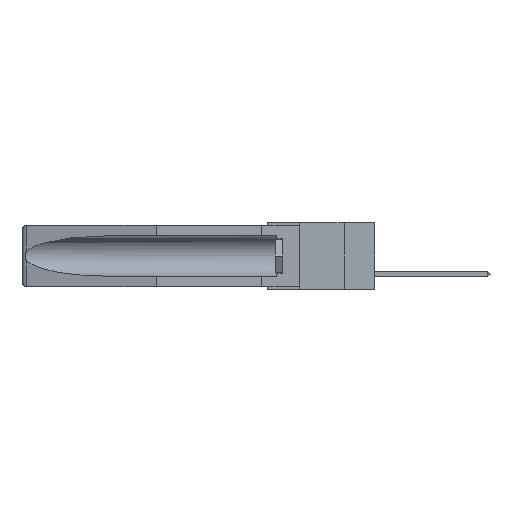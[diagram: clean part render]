
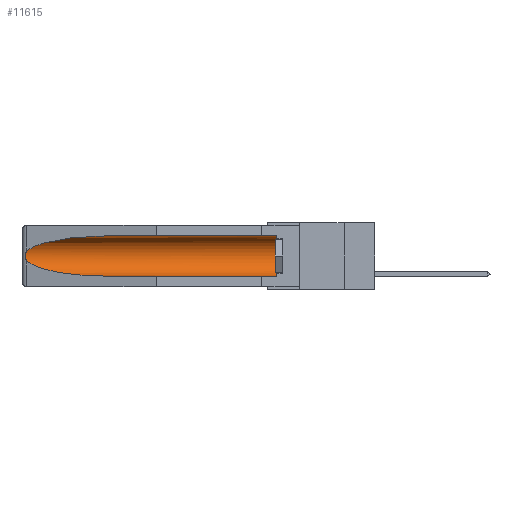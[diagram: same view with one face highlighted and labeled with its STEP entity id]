
A CAD part, left-side view. The second image highlights one B-rep face of the part: STEP entity #11615.
In plain terms, the highlighted cylindrical face has radius 2.857 mm (diameter 5.715 mm), a partial arc.
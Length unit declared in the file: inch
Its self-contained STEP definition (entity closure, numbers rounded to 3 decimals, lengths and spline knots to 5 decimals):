
#178 = AXIS2_PLACEMENT_3D ( 'NONE', #16693, #6734, #18355 ) ;
#640 = CARTESIAN_POINT ( 'NONE',  ( 0.26597, 1.5296, -0.19026 ) ) ;
#661 = CIRCLE ( 'NONE', #178, 0.1125 ) ;
#782 = CARTESIAN_POINT ( 'NONE',  ( 0.2673, 1.5327, -0.16383 ) ) ;
#856 = CARTESIAN_POINT ( 'NONE',  ( 0.2673, 1.53269, -0.17917 ) ) ;
#1087 = VERTEX_POINT ( 'NONE', #21462 ) ;
#1698 = CARTESIAN_POINT ( 'NONE',  ( 0.25451, 1.48313, -0.09465 ) ) ;
#1726 = EDGE_CURVE ( 'NONE', #5221, #7642, #12775, .T. ) ;
#2313 = CARTESIAN_POINT ( 'NONE',  ( 0.26654, 1.53092, -0.15636 ) ) ;
#3153 = ORIENTED_EDGE ( 'NONE', *, *, #1726, .T. ) ;
#3278 = EDGE_CURVE ( 'NONE', #10712, #8736, #7595, .T. ) ;
#3390 = ORIENTED_EDGE ( 'NONE', *, *, #7000, .F. ) ;
#3676 = EDGE_LOOP ( 'NONE', ( #18862, #15747, #3153, #3390, #4925, #5742 ) ) ;
#3760 = CARTESIAN_POINT ( 'NONE',  ( 0.155, -0.30754, -0.059 ) ) ;
#4052 = CARTESIAN_POINT ( 'NONE',  ( 0.25451, 1.48313, -0.24835 ) ) ;
#4061 = CARTESIAN_POINT ( 'NONE',  ( 0.2675, 1.53308, -0.17534 ) ) ;
#4267 = CARTESIAN_POINT ( 'NONE',  ( 0.21114, 1.30732, -0.284 ) ) ;
#4635 = EDGE_CURVE ( 'NONE', #11407, #1087, #661, .T. ) ;
#4812 = CARTESIAN_POINT ( 'NONE',  ( 0.26537, 1.52718, -0.14972 ) ) ;
#4925 = ORIENTED_EDGE ( 'NONE', *, *, #4635, .T. ) ;
#4960 = CARTESIAN_POINT ( 'NONE',  ( 0.21114, 1.30732, -0.059 ) ) ;
#5138 = LINE ( 'NONE', #3760, #9314 ) ;
#5221 = VERTEX_POINT ( 'NONE', #18161 ) ;
#5679 = CARTESIAN_POINT ( 'NONE',  ( 0.26537, 1.52718, -0.14972 ) ) ;
#5742 = ORIENTED_EDGE ( 'NONE', *, *, #10037, .T. ) ;
#5753 = CARTESIAN_POINT ( 'NONE',  ( 0.155, 0.126, -0.284 ) ) ;
#6734 = DIRECTION ( 'NONE',  ( 0., -1., 0. ) ) ;
#7000 = EDGE_CURVE ( 'NONE', #11407, #7642, #16149, .T. ) ;
#7356 = EDGE_CURVE ( 'NONE', #8736, #5221, #19863, .T. ) ;
#7595 =( BOUNDED_CURVE ( )  B_SPLINE_CURVE ( 3, ( #15014, #4960, #1698, #4812 ),
 .UNSPECIFIED., .F., .F. ) 
 B_SPLINE_CURVE_WITH_KNOTS ( ( 4, 4 ),
 ( 4.71239, 6.08839 ),
 .UNSPECIFIED. ) 
 CURVE ( )  GEOMETRIC_REPRESENTATION_ITEM ( )  RATIONAL_B_SPLINE_CURVE ( ( 1., 0.848, 0.848, 1. ) ) 
 REPRESENTATION_ITEM ( '' )  );
#7642 = VERTEX_POINT ( 'NONE', #20107 ) ;
#7922 = DIRECTION ( 'NONE',  ( 0., 0., 1. ) ) ;
#8483 = CYLINDRICAL_SURFACE ( 'NONE', #9733, 0.1125 ) ;
#8736 = VERTEX_POINT ( 'NONE', #5679 ) ;
#8780 = DIRECTION ( 'NONE',  ( 0., 1., 0. ) ) ;
#8874 = CARTESIAN_POINT ( 'NONE',  ( 0.26597, 1.52961, -0.15275 ) ) ;
#9314 = VECTOR ( 'NONE', #8780, 39.37008 ) ;
#9458 = DIRECTION ( 'NONE',  ( 0., 1., 0. ) ) ;
#9733 = AXIS2_PLACEMENT_3D ( 'NONE', #17867, #21228, #7922 ) ;
#10037 = EDGE_CURVE ( 'NONE', #1087, #10712, #5138, .T. ) ;
#10284 = FACE_OUTER_BOUND ( 'NONE', #3676, .T. ) ;
#10595 = CARTESIAN_POINT ( 'NONE',  ( 0.2675, 1.53308, -0.16763 ) ) ;
#10712 = VERTEX_POINT ( 'NONE', #12003 ) ;
#10804 = CARTESIAN_POINT ( 'NONE',  ( 0.26655, 1.53094, -0.18657 ) ) ;
#10825 = CARTESIAN_POINT ( 'NONE',  ( 0.155, -0.30754, -0.284 ) ) ;
#11407 = VERTEX_POINT ( 'NONE', #5753 ) ;
#11615 = ADVANCED_FACE ( 'NONE', ( #10284 ), #8483, .F. ) ;
#12003 = CARTESIAN_POINT ( 'NONE',  ( 0.155, 1.07973, -0.059 ) ) ;
#12764 = VECTOR ( 'NONE', #9458, 39.37008 ) ;
#12775 =( BOUNDED_CURVE ( )  B_SPLINE_CURVE ( 3, ( #17560, #4052, #4267, #17348 ),
 .UNSPECIFIED., .F., .T. ) 
 B_SPLINE_CURVE_WITH_KNOTS ( ( 4, 4 ),
 ( 0.1948, 1.5708 ),
 .UNSPECIFIED. ) 
 CURVE ( )  GEOMETRIC_REPRESENTATION_ITEM ( )  RATIONAL_B_SPLINE_CURVE ( ( 1., 0.848, 0.848, 1. ) ) 
 REPRESENTATION_ITEM ( '' )  );
#14088 = CARTESIAN_POINT ( 'NONE',  ( 0.26537, 1.52718, -0.19328 ) ) ;
#15014 = CARTESIAN_POINT ( 'NONE',  ( 0.155, 1.07973, -0.059 ) ) ;
#15641 = CARTESIAN_POINT ( 'NONE',  ( 0.26537, 1.52718, -0.14972 ) ) ;
#15747 = ORIENTED_EDGE ( 'NONE', *, *, #7356, .T. ) ;
#16149 = LINE ( 'NONE', #10825, #12764 ) ;
#16693 = CARTESIAN_POINT ( 'NONE',  ( 0.155, 0.126, -0.1715 ) ) ;
#17348 = CARTESIAN_POINT ( 'NONE',  ( 0.155, 1.07973, -0.284 ) ) ;
#17560 = CARTESIAN_POINT ( 'NONE',  ( 0.26537, 1.52718, -0.19328 ) ) ;
#17867 = CARTESIAN_POINT ( 'NONE',  ( 0.155, -0.30754, -0.1715 ) ) ;
#18161 = CARTESIAN_POINT ( 'NONE',  ( 0.26537, 1.52718, -0.19328 ) ) ;
#18355 = DIRECTION ( 'NONE',  ( 0., 0., 1. ) ) ;
#18862 = ORIENTED_EDGE ( 'NONE', *, *, #3278, .T. ) ;
#19863 = B_SPLINE_CURVE_WITH_KNOTS ( 'NONE', 3,
 ( #15641, #8874, #2313, #782, #10595, #4061, #856, #10804, #640, #14088 ),
 .UNSPECIFIED., .F., .F.,
 ( 4, 2, 2, 2, 4 ),
 ( 0., 0.00029, 0.00058, 0.00087, 0.00117 ),
 .UNSPECIFIED. ) ;
#20107 = CARTESIAN_POINT ( 'NONE',  ( 0.155, 1.07973, -0.284 ) ) ;
#21228 = DIRECTION ( 'NONE',  ( 0., 1., 0. ) ) ;
#21462 = CARTESIAN_POINT ( 'NONE',  ( 0.155, 0.126, -0.059 ) ) ;
